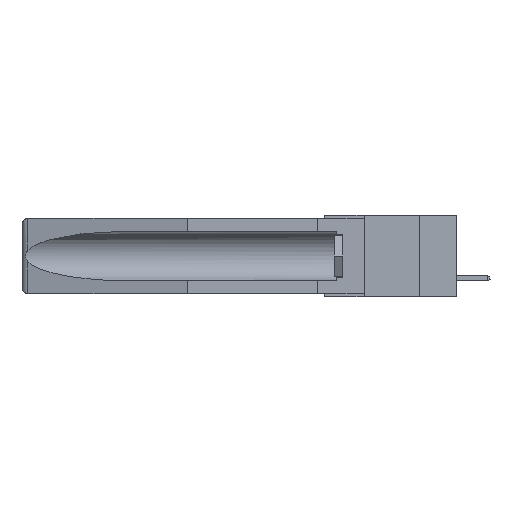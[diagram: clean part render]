
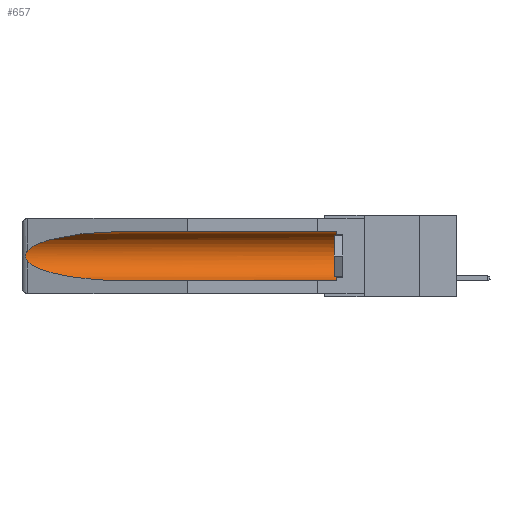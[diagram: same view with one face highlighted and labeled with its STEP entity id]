
A CAD part, left-side view. The second image highlights one B-rep face of the part: STEP entity #657.
In plain terms, the highlighted cylindrical face has radius 2.857 mm (diameter 5.715 mm), a partial arc.
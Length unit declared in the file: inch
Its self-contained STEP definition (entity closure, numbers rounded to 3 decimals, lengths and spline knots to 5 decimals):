
#657 = ADVANCED_FACE ( 'NONE', ( #24202 ), #1975, .F. ) ;
#1483 = ORIENTED_EDGE ( 'NONE', *, *, #2837, .T. ) ;
#1975 = CYLINDRICAL_SURFACE ( 'NONE', #3241, 0.1125 ) ;
#2347 = CARTESIAN_POINT ( 'NONE',  ( 0.155, 0.126, -0.059 ) ) ;
#2678 = DIRECTION ( 'NONE',  ( 0., 0., 1. ) ) ;
#2697 = CARTESIAN_POINT ( 'NONE',  ( 0.2673, 1.5327, -0.16383 ) ) ;
#2837 = EDGE_CURVE ( 'NONE', #12334, #17777, #24750, .T. ) ;
#2866 = CARTESIAN_POINT ( 'NONE',  ( 0.26537, 1.52718, -0.14972 ) ) ;
#3241 = AXIS2_PLACEMENT_3D ( 'NONE', #4309, #23844, #2678 ) ;
#4309 = CARTESIAN_POINT ( 'NONE',  ( 0.155, -0.30754, -0.1715 ) ) ;
#4791 = CARTESIAN_POINT ( 'NONE',  ( 0.26537, 1.52718, -0.14972 ) ) ;
#5288 = VERTEX_POINT ( 'NONE', #23051 ) ;
#6622 = VERTEX_POINT ( 'NONE', #2347 ) ;
#7159 = EDGE_LOOP ( 'NONE', ( #10450, #14429, #1483, #21562, #15344, #8944 ) ) ;
#7562 = CARTESIAN_POINT ( 'NONE',  ( 0.26537, 1.52718, -0.14972 ) ) ;
#7600 = EDGE_CURVE ( 'NONE', #14782, #16094, #15639, .T. ) ;
#7690 = LINE ( 'NONE', #14143, #10971 ) ;
#7783 = EDGE_CURVE ( 'NONE', #5288, #6622, #7820, .T. ) ;
#7820 = CIRCLE ( 'NONE', #13225, 0.1125 ) ;
#8584 = CARTESIAN_POINT ( 'NONE',  ( 0.25451, 1.48313, -0.09465 ) ) ;
#8944 = ORIENTED_EDGE ( 'NONE', *, *, #13135, .T. ) ;
#9876 = CARTESIAN_POINT ( 'NONE',  ( 0.26655, 1.53094, -0.18657 ) ) ;
#9944 = CARTESIAN_POINT ( 'NONE',  ( 0.25451, 1.48313, -0.24835 ) ) ;
#10044 = CARTESIAN_POINT ( 'NONE',  ( 0.26597, 1.5296, -0.19026 ) ) ;
#10450 = ORIENTED_EDGE ( 'NONE', *, *, #7600, .T. ) ;
#10473 = CARTESIAN_POINT ( 'NONE',  ( 0.26537, 1.52718, -0.19328 ) ) ;
#10971 = VECTOR ( 'NONE', #11940, 39.37008 ) ;
#11913 = DIRECTION ( 'NONE',  ( 0., 1., 0. ) ) ;
#11940 = DIRECTION ( 'NONE',  ( 0., 1., 0. ) ) ;
#12046 = CARTESIAN_POINT ( 'NONE',  ( 0.21114, 1.30732, -0.284 ) ) ;
#12134 = CARTESIAN_POINT ( 'NONE',  ( 0.26537, 1.52718, -0.19328 ) ) ;
#12334 = VERTEX_POINT ( 'NONE', #17359 ) ;
#12621 = CARTESIAN_POINT ( 'NONE',  ( 0.21114, 1.30732, -0.059 ) ) ;
#13135 = EDGE_CURVE ( 'NONE', #6622, #14782, #7690, .T. ) ;
#13206 = CARTESIAN_POINT ( 'NONE',  ( 0.155, 1.07973, -0.284 ) ) ;
#13225 = AXIS2_PLACEMENT_3D ( 'NONE', #19205, #25182, #21336 ) ;
#14143 = CARTESIAN_POINT ( 'NONE',  ( 0.155, -0.30754, -0.059 ) ) ;
#14429 = ORIENTED_EDGE ( 'NONE', *, *, #18585, .T. ) ;
#14782 = VERTEX_POINT ( 'NONE', #19345 ) ;
#15344 = ORIENTED_EDGE ( 'NONE', *, *, #7783, .T. ) ;
#15639 =( BOUNDED_CURVE ( )  B_SPLINE_CURVE ( 3, ( #16472, #12621, #8584, #4791 ),
 .UNSPECIFIED., .F., .F. ) 
 B_SPLINE_CURVE_WITH_KNOTS ( ( 4, 4 ),
 ( 4.71239, 6.08839 ),
 .UNSPECIFIED. ) 
 CURVE ( )  GEOMETRIC_REPRESENTATION_ITEM ( )  RATIONAL_B_SPLINE_CURVE ( ( 1., 0.848, 0.848, 1. ) ) 
 REPRESENTATION_ITEM ( '' )  );
#15804 = CARTESIAN_POINT ( 'NONE',  ( 0.155, 1.07973, -0.284 ) ) ;
#16094 = VERTEX_POINT ( 'NONE', #7562 ) ;
#16248 = CARTESIAN_POINT ( 'NONE',  ( 0.2675, 1.53308, -0.17534 ) ) ;
#16472 = CARTESIAN_POINT ( 'NONE',  ( 0.155, 1.07973, -0.059 ) ) ;
#17359 = CARTESIAN_POINT ( 'NONE',  ( 0.26537, 1.52718, -0.19328 ) ) ;
#17777 = VERTEX_POINT ( 'NONE', #13206 ) ;
#18223 = VECTOR ( 'NONE', #11913, 39.37008 ) ;
#18585 = EDGE_CURVE ( 'NONE', #16094, #12334, #18952, .T. ) ;
#18952 = B_SPLINE_CURVE_WITH_KNOTS ( 'NONE', 3,
 ( #2866, #21559, #21719, #2697, #23687, #16248, #19751, #9876, #10044, #10473 ),
 .UNSPECIFIED., .F., .F.,
 ( 4, 2, 2, 2, 4 ),
 ( 0., 0.00029, 0.00058, 0.00087, 0.00117 ),
 .UNSPECIFIED. ) ;
#19205 = CARTESIAN_POINT ( 'NONE',  ( 0.155, 0.126, -0.1715 ) ) ;
#19345 = CARTESIAN_POINT ( 'NONE',  ( 0.155, 1.07973, -0.059 ) ) ;
#19447 = LINE ( 'NONE', #19771, #18223 ) ;
#19751 = CARTESIAN_POINT ( 'NONE',  ( 0.2673, 1.53269, -0.17917 ) ) ;
#19771 = CARTESIAN_POINT ( 'NONE',  ( 0.155, -0.30754, -0.284 ) ) ;
#21336 = DIRECTION ( 'NONE',  ( 0., 0., 1. ) ) ;
#21559 = CARTESIAN_POINT ( 'NONE',  ( 0.26597, 1.52961, -0.15275 ) ) ;
#21562 = ORIENTED_EDGE ( 'NONE', *, *, #24176, .F. ) ;
#21719 = CARTESIAN_POINT ( 'NONE',  ( 0.26654, 1.53092, -0.15636 ) ) ;
#23051 = CARTESIAN_POINT ( 'NONE',  ( 0.155, 0.126, -0.284 ) ) ;
#23687 = CARTESIAN_POINT ( 'NONE',  ( 0.2675, 1.53308, -0.16763 ) ) ;
#23844 = DIRECTION ( 'NONE',  ( 0., 1., 0. ) ) ;
#24176 = EDGE_CURVE ( 'NONE', #5288, #17777, #19447, .T. ) ;
#24202 = FACE_OUTER_BOUND ( 'NONE', #7159, .T. ) ;
#24750 =( BOUNDED_CURVE ( )  B_SPLINE_CURVE ( 3, ( #12134, #9944, #12046, #15804 ),
 .UNSPECIFIED., .F., .F. ) 
 B_SPLINE_CURVE_WITH_KNOTS ( ( 4, 4 ),
 ( 0.1948, 1.5708 ),
 .UNSPECIFIED. ) 
 CURVE ( )  GEOMETRIC_REPRESENTATION_ITEM ( )  RATIONAL_B_SPLINE_CURVE ( ( 1., 0.848, 0.848, 1. ) ) 
 REPRESENTATION_ITEM ( '' )  );
#25182 = DIRECTION ( 'NONE',  ( 0., -1., 0. ) ) ;
